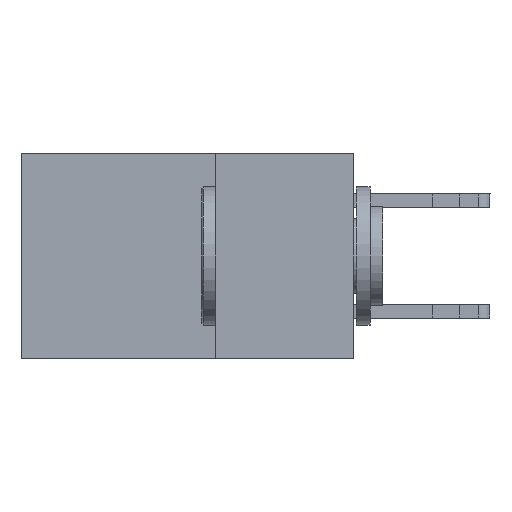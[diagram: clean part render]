
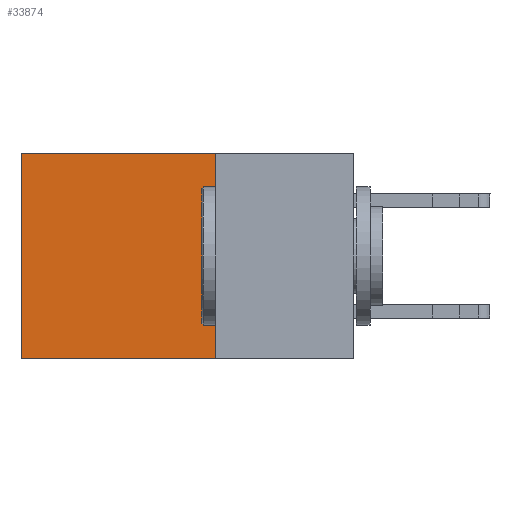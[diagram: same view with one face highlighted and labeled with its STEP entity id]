
A CAD part, left-side view. The second image highlights one B-rep face of the part: STEP entity #33874.
In plain terms, the highlighted planar face has unit normal (-1, 0, 0).
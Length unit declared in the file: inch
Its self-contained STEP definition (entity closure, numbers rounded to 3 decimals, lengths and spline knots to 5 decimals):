
#456 = ORIENTED_EDGE ( 'NONE', *, *, #26035, .T. ) ;
#590 = ORIENTED_EDGE ( 'NONE', *, *, #9658, .F. ) ;
#1135 = VERTEX_POINT ( 'NONE', #17886 ) ;
#4155 = VECTOR ( 'NONE', #9430, 39.37008 ) ;
#5110 = LINE ( 'NONE', #5764, #28118 ) ;
#5764 = CARTESIAN_POINT ( 'NONE',  ( 0.2875, 0.25, 0. ) ) ;
#7751 = PLANE ( 'NONE',  #15018 ) ;
#9010 = EDGE_LOOP ( 'NONE', ( #29597, #590, #33125, #456 ) ) ;
#9430 = DIRECTION ( 'NONE',  ( 0., 1., 0. ) ) ;
#9658 = EDGE_CURVE ( 'NONE', #32664, #15793, #36785, .T. ) ;
#14275 = EDGE_CURVE ( 'NONE', #36297, #15793, #22612, .T. ) ;
#15018 = AXIS2_PLACEMENT_3D ( 'NONE', #28364, #16520, #37156 ) ;
#15793 = VERTEX_POINT ( 'NONE', #24189 ) ;
#16520 = DIRECTION ( 'NONE',  ( 1., 0., 0. ) ) ;
#17886 = CARTESIAN_POINT ( 'NONE',  ( 0.2875, 0.25, 0. ) ) ;
#18869 = VECTOR ( 'NONE', #36729, 39.37008 ) ;
#20723 = DIRECTION ( 'NONE',  ( 0., 1., 0. ) ) ;
#21040 = FACE_OUTER_BOUND ( 'NONE', #9010, .T. ) ;
#21917 = CARTESIAN_POINT ( 'NONE',  ( 0.2875, 0.6, 0. ) ) ;
#22612 = LINE ( 'NONE', #28587, #18869 ) ;
#24189 = CARTESIAN_POINT ( 'NONE',  ( 0.2875, 0.6, -0.37 ) ) ;
#24703 = EDGE_CURVE ( 'NONE', #1135, #32664, #26817, .T. ) ;
#25904 = VECTOR ( 'NONE', #31195, 39.37008 ) ;
#26035 = EDGE_CURVE ( 'NONE', #1135, #36297, #5110, .T. ) ;
#26817 = LINE ( 'NONE', #30925, #25904 ) ;
#28118 = VECTOR ( 'NONE', #20723, 39.37008 ) ;
#28364 = CARTESIAN_POINT ( 'NONE',  ( 0.2875, 0.25, 0. ) ) ;
#28587 = CARTESIAN_POINT ( 'NONE',  ( 0.2875, 0.6, 0. ) ) ;
#29597 = ORIENTED_EDGE ( 'NONE', *, *, #14275, .T. ) ;
#30159 = CARTESIAN_POINT ( 'NONE',  ( 0.2875, 0.25, -0.37 ) ) ;
#30925 = CARTESIAN_POINT ( 'NONE',  ( 0.2875, 0.25, 0. ) ) ;
#31195 = DIRECTION ( 'NONE',  ( 0., 0., -1. ) ) ;
#32664 = VERTEX_POINT ( 'NONE', #37918 ) ;
#33125 = ORIENTED_EDGE ( 'NONE', *, *, #24703, .F. ) ;
#33874 = ADVANCED_FACE ( 'NONE', ( #21040 ), #7751, .F. ) ;
#36297 = VERTEX_POINT ( 'NONE', #21917 ) ;
#36729 = DIRECTION ( 'NONE',  ( 0., 0., -1. ) ) ;
#36785 = LINE ( 'NONE', #30159, #4155 ) ;
#37156 = DIRECTION ( 'NONE',  ( 0., 0., -1. ) ) ;
#37918 = CARTESIAN_POINT ( 'NONE',  ( 0.2875, 0.25, -0.37 ) ) ;
